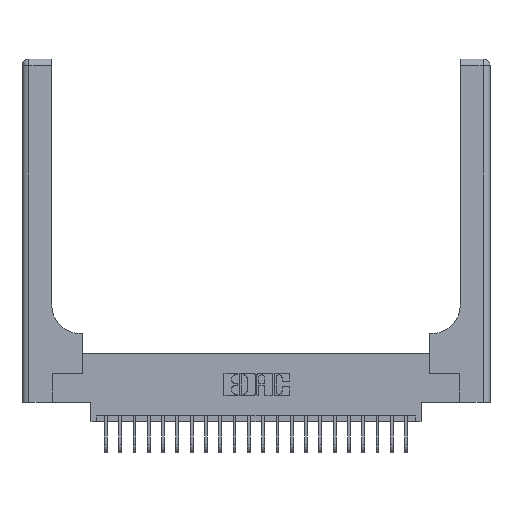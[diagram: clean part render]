
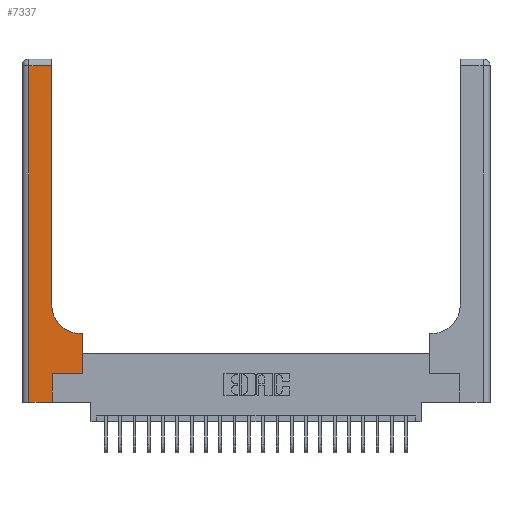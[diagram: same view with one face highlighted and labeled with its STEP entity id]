
A CAD part, top view. The second image highlights one B-rep face of the part: STEP entity #7337.
In plain terms, the highlighted planar face has unit normal (0, 0, 1).
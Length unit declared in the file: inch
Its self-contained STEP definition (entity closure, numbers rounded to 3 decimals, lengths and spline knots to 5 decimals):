
#96 = EDGE_CURVE ( 'NONE', #3493, #5811, #7805, .T. ) ;
#626 = DIRECTION ( 'NONE',  ( -1., 0., 0. ) ) ;
#1433 = CARTESIAN_POINT ( 'NONE',  ( 0.265, 0., 0.37 ) ) ;
#1490 = EDGE_CURVE ( 'NONE', #11143, #12509, #5469, .T. ) ;
#1506 = LINE ( 'NONE', #13162, #12812 ) ;
#2210 = LINE ( 'NONE', #19374, #14701 ) ;
#2358 = VERTEX_POINT ( 'NONE', #18971 ) ;
#3215 = DIRECTION ( 'NONE',  ( 1., 0., 0. ) ) ;
#3493 = VERTEX_POINT ( 'NONE', #3636 ) ;
#3636 = CARTESIAN_POINT ( 'NONE',  ( 0.51, 0.6, 0.37 ) ) ;
#3775 = EDGE_LOOP ( 'NONE', ( #17722, #19714, #16419, #6063, #8946, #20993, #18163, #4946, #5592 ) ) ;
#3941 = FACE_OUTER_BOUND ( 'NONE', #3775, .T. ) ;
#4231 = DIRECTION ( 'NONE',  ( 0., 1., 0. ) ) ;
#4242 = VECTOR ( 'NONE', #16436, 39.37008 ) ;
#4276 = DIRECTION ( 'NONE',  ( 0., 0., -1. ) ) ;
#4353 = DIRECTION ( 'NONE',  ( 0., 0., -1. ) ) ;
#4946 = ORIENTED_EDGE ( 'NONE', *, *, #17284, .T. ) ;
#5469 = LINE ( 'NONE', #17791, #10895 ) ;
#5592 = ORIENTED_EDGE ( 'NONE', *, *, #96, .T. ) ;
#5811 = VERTEX_POINT ( 'NONE', #11695 ) ;
#6035 = CARTESIAN_POINT ( 'NONE',  ( 0.51, 0.85, 0.37 ) ) ;
#6063 = ORIENTED_EDGE ( 'NONE', *, *, #12029, .T. ) ;
#6149 = CARTESIAN_POINT ( 'NONE',  ( 0.528, 0.25, 0.37 ) ) ;
#6259 = LINE ( 'NONE', #6149, #19915 ) ;
#7337 = ADVANCED_FACE ( 'NONE', ( #3941 ), #7517, .F. ) ;
#7411 = CARTESIAN_POINT ( 'NONE',  ( 0., 3., 0.37 ) ) ;
#7517 = PLANE ( 'NONE',  #15952 ) ;
#7660 = CARTESIAN_POINT ( 'NONE',  ( 0.26, 2.94, 0.37 ) ) ;
#7773 = CARTESIAN_POINT ( 'NONE',  ( 0.06, 2.94, 0.37 ) ) ;
#7805 = CIRCLE ( 'NONE', #8506, 0.25 ) ;
#7887 = EDGE_CURVE ( 'NONE', #8756, #17028, #6259, .T. ) ;
#8458 = DIRECTION ( 'NONE',  ( 0., 1., 0. ) ) ;
#8506 = AXIS2_PLACEMENT_3D ( 'NONE', #6035, #4353, #3215 ) ;
#8756 = VERTEX_POINT ( 'NONE', #8852 ) ;
#8852 = CARTESIAN_POINT ( 'NONE',  ( 0.528, 0.25, 0.37 ) ) ;
#8946 = ORIENTED_EDGE ( 'NONE', *, *, #14923, .T. ) ;
#10185 = VERTEX_POINT ( 'NONE', #18711 ) ;
#10436 = EDGE_CURVE ( 'NONE', #12509, #2358, #1506, .T. ) ;
#10895 = VECTOR ( 'NONE', #626, 39.37008 ) ;
#11143 = VERTEX_POINT ( 'NONE', #7660 ) ;
#11472 = CARTESIAN_POINT ( 'NONE',  ( 0., 0., 0.37 ) ) ;
#11695 = CARTESIAN_POINT ( 'NONE',  ( 0.26, 0.85, 0.37 ) ) ;
#12029 = EDGE_CURVE ( 'NONE', #2358, #20439, #20145, .T. ) ;
#12193 = VECTOR ( 'NONE', #12406, 39.37008 ) ;
#12406 = DIRECTION ( 'NONE',  ( -1., 0., 0. ) ) ;
#12509 = VERTEX_POINT ( 'NONE', #7773 ) ;
#12812 = VECTOR ( 'NONE', #14958, 39.37008 ) ;
#13162 = CARTESIAN_POINT ( 'NONE',  ( 0.06, 3., 0.37 ) ) ;
#14701 = VECTOR ( 'NONE', #4231, 39.37008 ) ;
#14923 = EDGE_CURVE ( 'NONE', #20439, #10185, #2210, .T. ) ;
#14958 = DIRECTION ( 'NONE',  ( 0., -1., 0. ) ) ;
#15288 = LINE ( 'NONE', #22139, #17617 ) ;
#15952 = AXIS2_PLACEMENT_3D ( 'NONE', #7411, #4276, #20996 ) ;
#16194 = VECTOR ( 'NONE', #18762, 39.37008 ) ;
#16283 = CARTESIAN_POINT ( 'NONE',  ( 0.528, 0.6, 0.37 ) ) ;
#16419 = ORIENTED_EDGE ( 'NONE', *, *, #10436, .T. ) ;
#16436 = DIRECTION ( 'NONE',  ( 1., 0., 0. ) ) ;
#16964 = LINE ( 'NONE', #20779, #16194 ) ;
#17028 = VERTEX_POINT ( 'NONE', #16283 ) ;
#17284 = EDGE_CURVE ( 'NONE', #17028, #3493, #19275, .T. ) ;
#17617 = VECTOR ( 'NONE', #20460, 39.37008 ) ;
#17722 = ORIENTED_EDGE ( 'NONE', *, *, #17912, .T. ) ;
#17791 = CARTESIAN_POINT ( 'NONE',  ( 0., 2.94, 0.37 ) ) ;
#17912 = EDGE_CURVE ( 'NONE', #5811, #11143, #15288, .T. ) ;
#18163 = ORIENTED_EDGE ( 'NONE', *, *, #7887, .T. ) ;
#18711 = CARTESIAN_POINT ( 'NONE',  ( 0.265, 0.25, 0.37 ) ) ;
#18762 = DIRECTION ( 'NONE',  ( 1., 0., 0. ) ) ;
#18971 = CARTESIAN_POINT ( 'NONE',  ( 0.06, 0., 0.37 ) ) ;
#19275 = LINE ( 'NONE', #21071, #12193 ) ;
#19374 = CARTESIAN_POINT ( 'NONE',  ( 0.265, 0., 0.37 ) ) ;
#19714 = ORIENTED_EDGE ( 'NONE', *, *, #1490, .T. ) ;
#19915 = VECTOR ( 'NONE', #8458, 39.37008 ) ;
#20145 = LINE ( 'NONE', #11472, #4242 ) ;
#20169 = EDGE_CURVE ( 'NONE', #10185, #8756, #16964, .T. ) ;
#20439 = VERTEX_POINT ( 'NONE', #1433 ) ;
#20460 = DIRECTION ( 'NONE',  ( 0., 1., 0. ) ) ;
#20779 = CARTESIAN_POINT ( 'NONE',  ( 0.265, 0.25, 0.37 ) ) ;
#20993 = ORIENTED_EDGE ( 'NONE', *, *, #20169, .T. ) ;
#20996 = DIRECTION ( 'NONE',  ( -1., 0., 0. ) ) ;
#21071 = CARTESIAN_POINT ( 'NONE',  ( 0.26, 0.6, 0.37 ) ) ;
#22139 = CARTESIAN_POINT ( 'NONE',  ( 0.26, 3., 0.37 ) ) ;
